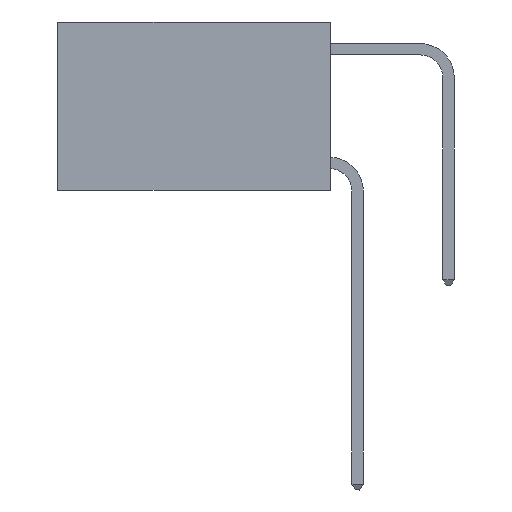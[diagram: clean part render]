
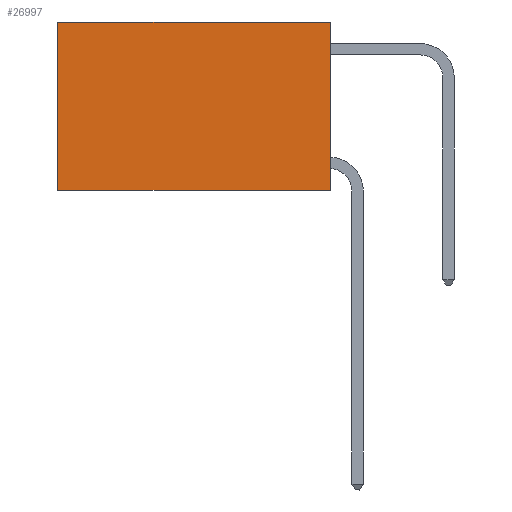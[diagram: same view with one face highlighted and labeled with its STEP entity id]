
A CAD part, left-side view. The second image highlights one B-rep face of the part: STEP entity #26997.
In plain terms, the highlighted planar face has unit normal (-1, 0, 0).
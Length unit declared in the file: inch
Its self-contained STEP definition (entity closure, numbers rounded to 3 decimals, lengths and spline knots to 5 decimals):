
#154 = VERTEX_POINT ( 'NONE', #22579 ) ;
#374 = CARTESIAN_POINT ( 'NONE',  ( 0.2625, 0., 0. ) ) ;
#793 = CARTESIAN_POINT ( 'NONE',  ( 0.2625, 0.6, 0. ) ) ;
#2100 = VECTOR ( 'NONE', #3073, 39.37008 ) ;
#3073 = DIRECTION ( 'NONE',  ( 0., 0., -1. ) ) ;
#3238 = VECTOR ( 'NONE', #21487, 39.37008 ) ;
#4039 = EDGE_CURVE ( 'NONE', #15348, #18789, #26882, .T. ) ;
#5993 = CARTESIAN_POINT ( 'NONE',  ( 0.2625, 0.6, 0. ) ) ;
#6153 = PLANE ( 'NONE',  #21148 ) ;
#6441 = EDGE_CURVE ( 'NONE', #18789, #154, #17866, .T. ) ;
#8450 = DIRECTION ( 'NONE',  ( 0., 0., -1. ) ) ;
#9473 = ORIENTED_EDGE ( 'NONE', *, *, #22323, .T. ) ;
#9512 = VERTEX_POINT ( 'NONE', #5993 ) ;
#10372 = ORIENTED_EDGE ( 'NONE', *, *, #23521, .T. ) ;
#13129 = DIRECTION ( 'NONE',  ( 0., 1., 0. ) ) ;
#13342 = EDGE_LOOP ( 'NONE', ( #10372, #15423, #23903, #9473 ) ) ;
#15348 = VERTEX_POINT ( 'NONE', #26195 ) ;
#15423 = ORIENTED_EDGE ( 'NONE', *, *, #6441, .F. ) ;
#17173 = VECTOR ( 'NONE', #13129, 39.37008 ) ;
#17866 = LINE ( 'NONE', #19873, #17173 ) ;
#18789 = VERTEX_POINT ( 'NONE', #20217 ) ;
#19194 = CARTESIAN_POINT ( 'NONE',  ( 0.2625, 0., 0. ) ) ;
#19873 = CARTESIAN_POINT ( 'NONE',  ( 0.2625, 0., -0.37 ) ) ;
#20217 = CARTESIAN_POINT ( 'NONE',  ( 0.2625, 0., -0.37 ) ) ;
#20300 = LINE ( 'NONE', #793, #2100 ) ;
#21148 = AXIS2_PLACEMENT_3D ( 'NONE', #21978, #22080, #8450 ) ;
#21444 = LINE ( 'NONE', #19194, #3238 ) ;
#21487 = DIRECTION ( 'NONE',  ( 0., 1., 0. ) ) ;
#21978 = CARTESIAN_POINT ( 'NONE',  ( 0.2625, 0., 0. ) ) ;
#22080 = DIRECTION ( 'NONE',  ( 1., 0., 0. ) ) ;
#22323 = EDGE_CURVE ( 'NONE', #15348, #9512, #21444, .T. ) ;
#22579 = CARTESIAN_POINT ( 'NONE',  ( 0.2625, 0.6, -0.37 ) ) ;
#23521 = EDGE_CURVE ( 'NONE', #9512, #154, #20300, .T. ) ;
#23903 = ORIENTED_EDGE ( 'NONE', *, *, #4039, .F. ) ;
#26195 = CARTESIAN_POINT ( 'NONE',  ( 0.2625, 0., 0. ) ) ;
#26199 = VECTOR ( 'NONE', #27635, 39.37008 ) ;
#26821 = FACE_OUTER_BOUND ( 'NONE', #13342, .T. ) ;
#26882 = LINE ( 'NONE', #374, #26199 ) ;
#26997 = ADVANCED_FACE ( 'NONE', ( #26821 ), #6153, .F. ) ;
#27635 = DIRECTION ( 'NONE',  ( 0., 0., -1. ) ) ;
